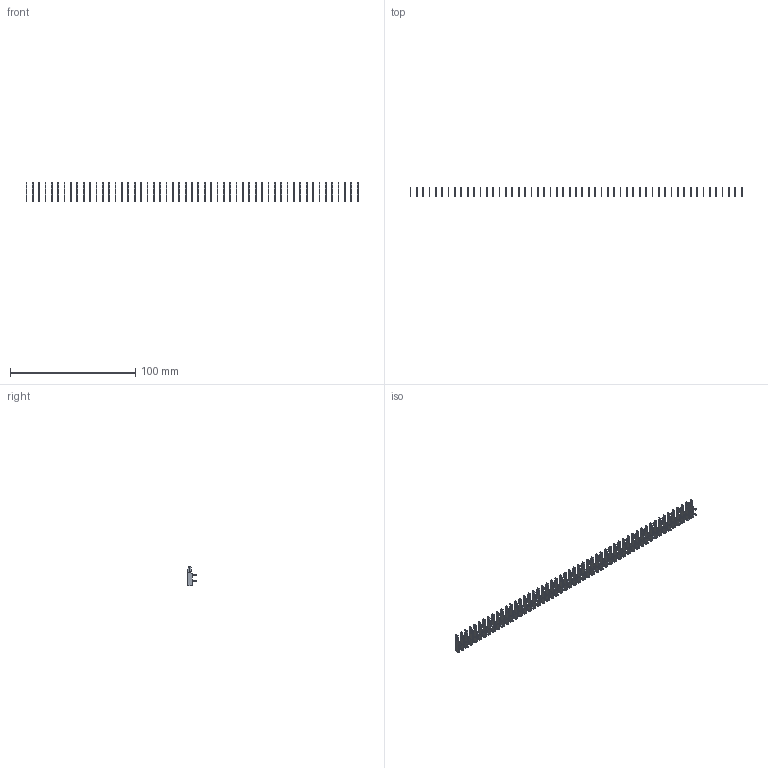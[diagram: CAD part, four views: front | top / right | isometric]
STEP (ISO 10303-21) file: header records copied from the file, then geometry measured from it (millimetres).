
FILE_DESCRIPTION (( 'STEP AP203' ), '1' );
FILE_NAME ('105-053-202-200.STEP', '2020-04-08T00:34:32', ( '' ), ( '' ), 'SwSTEP 2.0', 'SolidWorks 2016', '' );
FILE_SCHEMA (( 'CONFIG_CONTROL_DESIGN' ));
Length unit declared in the file: inch
Products named in the file (2): 100-290-001_100-290-202; 105-053-202-200
Assembly tree (53 placements, depth 2):
  105-053-202-200
    100-290-001_100-290-202  x53
Bounding box: 264.76 x 6.53 x 15.88 mm (x, y, z)
Volume: 1683.9 mm3; surface area: 7488.9 mm2
Topology: 53 solids, 53 shells, 1590 faces, 4452 edges, 2968 vertices
Faces by surface type: plane 1219, cylinder 371
Entity records: 2826 total; most frequent: DIRECTION 266, CARTESIAN_POINT 238, ORIENTED_EDGE 168, LOCAL_TIME 116, CALENDAR_DATE 116, COORDINATED_UNIVERSAL_TIME_OFFSET 116, DATE_AND_TIME 116, AXIS2_PLACEMENT_3D 100
